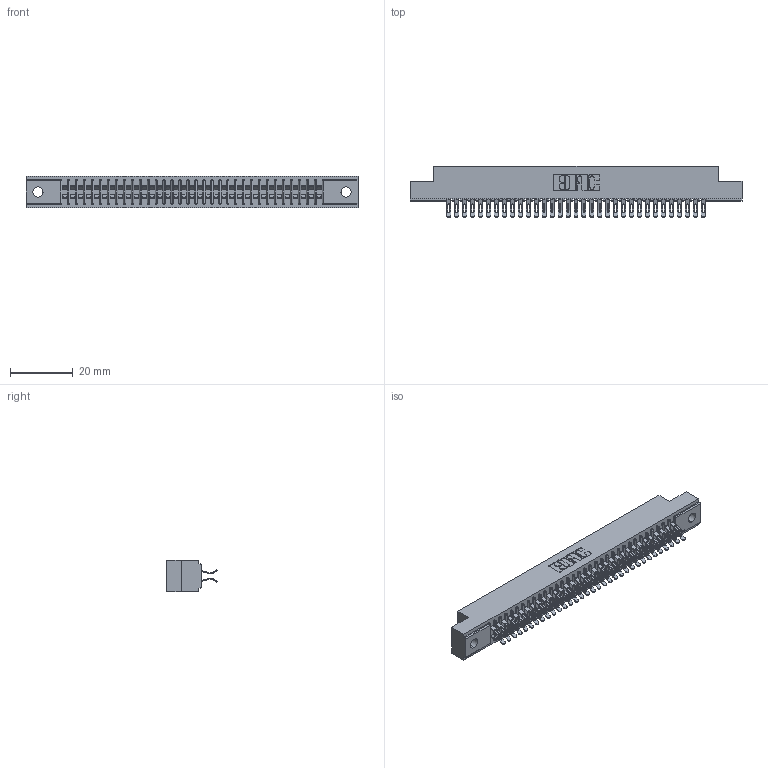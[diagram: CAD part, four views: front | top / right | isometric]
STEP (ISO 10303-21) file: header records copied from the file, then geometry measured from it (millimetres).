
FILE_DESCRIPTION (( 'STEP AP203' ), '1' );
FILE_NAME ('391-066-555-202.STEP', '2018-08-09T13:32:53', ( '' ), ( '' ), 'SwSTEP 2.0', 'SolidWorks 2016', '' );
FILE_SCHEMA (( 'CONFIG_CONTROL_DESIGN' ));
Length unit declared in the file: inch
Products named in the file (3): 341 Part_.128 (3.25) Dia Mounting Holes; 341-292-001_341-292-155; 391-066-555-202
Assembly tree (67 placements, depth 2):
  391-066-555-202
    341 Part_.128 (3.25) Dia Mounting Holes
    341-292-001_341-292-155  x66
Bounding box: 106.05 x 16.31 x 10.16 mm (x, y, z)
Volume: 7866.7 mm3; surface area: 13968.1 mm2
Topology: 67 solids, 67 shells, 5264 faces, 15727 edges, 10238 vertices
Faces by surface type: plane 2840, cylinder 2292, sphere 68, torus 64
Entity records: 41608 total; most frequent: CARTESIAN_POINT 6933, ORIENTED_EDGE 6878, DIRECTION 6725, EDGE_CURVE 3439, LINE 2753, VECTOR 2753, VERTEX_POINT 2178, AXIS2_PLACEMENT_3D 1986
